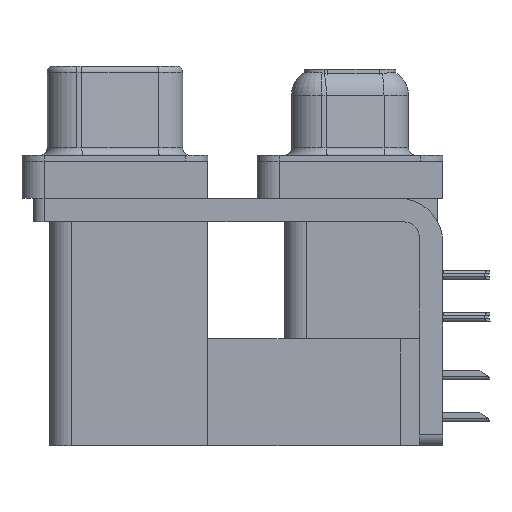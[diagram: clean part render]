
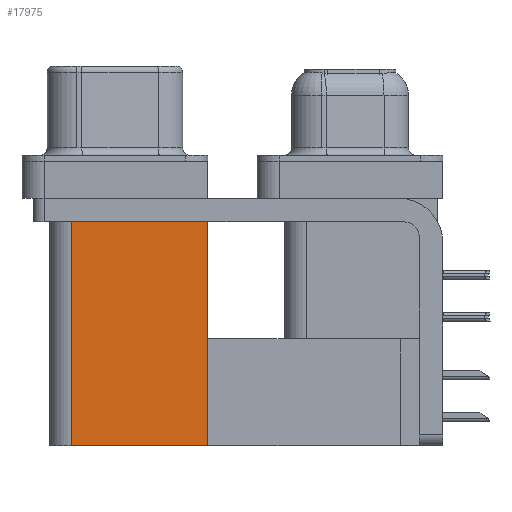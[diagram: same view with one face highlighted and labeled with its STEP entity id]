
A CAD part, left-side view. The second image highlights one B-rep face of the part: STEP entity #17975.
In plain terms, the highlighted planar face has unit normal (-1, 0, 0).
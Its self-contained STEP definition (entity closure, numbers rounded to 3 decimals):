
#1997 = CARTESIAN_POINT ( 'NONE',  ( 3.765, 18.8, -19.2 ) ) ;
#2981 = ORIENTED_EDGE ( 'NONE', *, *, #22556, .F. ) ;
#6715 = CARTESIAN_POINT ( 'NONE',  ( 3.765, 9.6, -19.2 ) ) ;
#8534 = DIRECTION ( 'NONE',  ( 0., 1., 0. ) ) ;
#9632 = VERTEX_POINT ( 'NONE', #22001 ) ;
#12102 = CARTESIAN_POINT ( 'NONE',  ( 3.765, 9.6, -19.2 ) ) ;
#17160 = EDGE_LOOP ( 'NONE', ( #24795, #2981, #37961, #33356 ) ) ;
#17299 = VECTOR ( 'NONE', #22131, 1000. ) ;
#17970 = CARTESIAN_POINT ( 'NONE',  ( 3.765, 9.6, -19.2 ) ) ;
#17975 = ADVANCED_FACE ( 'NONE', ( #40752 ), #37417, .F. ) ;
#18591 = AXIS2_PLACEMENT_3D ( 'NONE', #6715, #34289, #40971 ) ;
#21751 = EDGE_CURVE ( 'NONE', #28457, #31963, #41527, .T. ) ;
#22001 = CARTESIAN_POINT ( 'NONE',  ( 3.765, 18.8, -19.2 ) ) ;
#22131 = DIRECTION ( 'NONE',  ( 0., 1., 0. ) ) ;
#22556 = EDGE_CURVE ( 'NONE', #9632, #31963, #39164, .T. ) ;
#23325 = CARTESIAN_POINT ( 'NONE',  ( 3.765, 18.8, -2.5 ) ) ;
#24795 = ORIENTED_EDGE ( 'NONE', *, *, #21751, .T. ) ;
#28394 = DIRECTION ( 'NONE',  ( 0., 0., 1. ) ) ;
#28457 = VERTEX_POINT ( 'NONE', #32578 ) ;
#30289 = VECTOR ( 'NONE', #36251, 1000. ) ;
#31521 = VERTEX_POINT ( 'NONE', #38590 ) ;
#31901 = CARTESIAN_POINT ( 'NONE',  ( 3.765, 9.6, -2.5 ) ) ;
#31963 = VERTEX_POINT ( 'NONE', #23325 ) ;
#32578 = CARTESIAN_POINT ( 'NONE',  ( 3.765, 9.6, -2.5 ) ) ;
#33356 = ORIENTED_EDGE ( 'NONE', *, *, #34634, .T. ) ;
#34289 = DIRECTION ( 'NONE',  ( 1., 0., 0. ) ) ;
#34634 = EDGE_CURVE ( 'NONE', #31521, #28457, #39097, .T. ) ;
#36251 = DIRECTION ( 'NONE',  ( 0., 0., 1. ) ) ;
#36312 = VECTOR ( 'NONE', #28394, 1000. ) ;
#37417 = PLANE ( 'NONE',  #18591 ) ;
#37785 = EDGE_CURVE ( 'NONE', #31521, #9632, #42409, .T. ) ;
#37961 = ORIENTED_EDGE ( 'NONE', *, *, #37785, .F. ) ;
#38590 = CARTESIAN_POINT ( 'NONE',  ( 3.765, 9.6, -19.2 ) ) ;
#39097 = LINE ( 'NONE', #17970, #36312 ) ;
#39164 = LINE ( 'NONE', #1997, #30289 ) ;
#40752 = FACE_OUTER_BOUND ( 'NONE', #17160, .T. ) ;
#40959 = VECTOR ( 'NONE', #8534, 1000. ) ;
#40971 = DIRECTION ( 'NONE',  ( 0., 0., -1. ) ) ;
#41527 = LINE ( 'NONE', #31901, #40959 ) ;
#42409 = LINE ( 'NONE', #12102, #17299 ) ;
